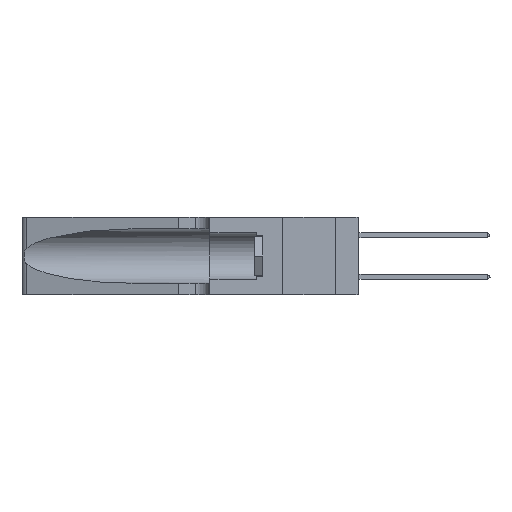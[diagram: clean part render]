
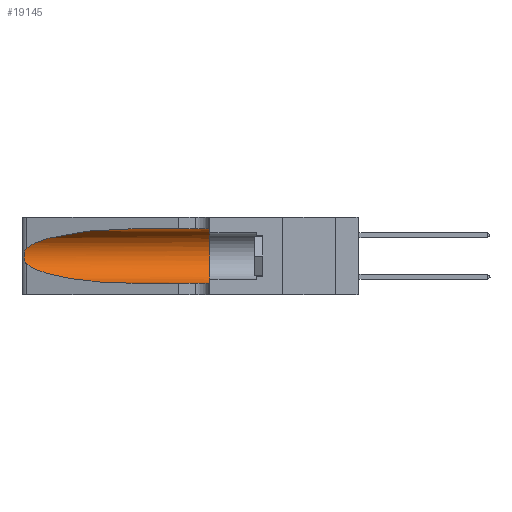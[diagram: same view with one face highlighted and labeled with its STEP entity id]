
A CAD part, left-side view. The second image highlights one B-rep face of the part: STEP entity #19145.
In plain terms, the highlighted cylindrical face has radius 3.308 mm (diameter 6.617 mm), a partial arc.
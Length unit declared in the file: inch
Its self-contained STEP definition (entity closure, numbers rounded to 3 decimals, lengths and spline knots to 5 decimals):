
#347 = EDGE_CURVE ( 'NONE', #3570, #11113, #22478, .T. ) ;
#1170 = CARTESIAN_POINT ( 'NONE',  ( 0.1305, 1.61858, 0.185 ) ) ;
#1408 = CARTESIAN_POINT ( 'NONE',  ( 0.1305, 0.72297, 0.05475 ) ) ;
#1459 = CIRCLE ( 'NONE', #18215, 0.13025 ) ;
#1961 = CARTESIAN_POINT ( 'NONE',  ( 0.25555, 1.22994, 0.2215 ) ) ;
#3570 = VERTEX_POINT ( 'NONE', #20307 ) ;
#3622 = DIRECTION ( 'NONE',  ( 0., -1., 0. ) ) ;
#4078 = DIRECTION ( 'NONE',  ( 0., 1., 0. ) ) ;
#4088 = CARTESIAN_POINT ( 'NONE',  ( 0.25787, 1.23484, 0.2124 ) ) ;
#4177 = CARTESIAN_POINT ( 'NONE',  ( 0.2373, 1.15595, 0.08982 ) ) ;
#4450 = CARTESIAN_POINT ( 'NONE',  ( 0.25639, 1.23186, 0.15144 ) ) ;
#4745 = CARTESIAN_POINT ( 'NONE',  ( 0.18966, 0.96281, 0.05475 ) ) ;
#5705 = CARTESIAN_POINT ( 'NONE',  ( 0.25487, 1.22718, 0.14631 ) ) ;
#5797 = ORIENTED_EDGE ( 'NONE', *, *, #26388, .T. ) ;
#5936 = ORIENTED_EDGE ( 'NONE', *, *, #347, .T. ) ;
#6123 = DIRECTION ( 'NONE',  ( 0., -1., 0. ) ) ;
#7045 = FACE_OUTER_BOUND ( 'NONE', #16669, .T. ) ;
#7656 = DIRECTION ( 'NONE',  ( 0., 0., -1. ) ) ;
#8499 = VERTEX_POINT ( 'NONE', #5705 ) ;
#8625 = CARTESIAN_POINT ( 'NONE',  ( 0.25555, 1.22993, 0.14849 ) ) ;
#8767 = CARTESIAN_POINT ( 'NONE',  ( 0.1305, 0.72297, 0.31525 ) ) ;
#9034 = CARTESIAN_POINT ( 'NONE',  ( 0.18966, 0.96281, 0.31525 ) ) ;
#9216 = ORIENTED_EDGE ( 'NONE', *, *, #14491, .T. ) ;
#10194 = CARTESIAN_POINT ( 'NONE',  ( 0.1305, 1.61858, 0.31525 ) ) ;
#10457 = ORIENTED_EDGE ( 'NONE', *, *, #23995, .F. ) ;
#10915 = CARTESIAN_POINT ( 'NONE',  ( 0.1305, 0.72297, 0.05475 ) ) ;
#11113 = VERTEX_POINT ( 'NONE', #25101 ) ;
#12879 = CARTESIAN_POINT ( 'NONE',  ( 0.26075, 1.23896, 0.19203 ) ) ;
#12976 = ORIENTED_EDGE ( 'NONE', *, *, #24922, .T. ) ;
#13323 = VERTEX_POINT ( 'NONE', #26771 ) ;
#13886 = VERTEX_POINT ( 'NONE', #10915 ) ;
#13900 = ORIENTED_EDGE ( 'NONE', *, *, #17628, .F. ) ;
#14491 = EDGE_CURVE ( 'NONE', #13886, #23960, #15539, .T. ) ;
#14859 = DIRECTION ( 'NONE',  ( 0., 0., 1. ) ) ;
#15539 = LINE ( 'NONE', #20869, #16569 ) ;
#16569 = VECTOR ( 'NONE', #3622, 39.37008 ) ;
#16669 = EDGE_LOOP ( 'NONE', ( #5936, #5797, #12976, #9216, #13900, #10457 ) ) ;
#16904 = CARTESIAN_POINT ( 'NONE',  ( 0.1305, 0.35, 0.05475 ) ) ;
#17628 = EDGE_CURVE ( 'NONE', #13323, #23960, #1459, .T. ) ;
#17926 = VECTOR ( 'NONE', #6123, 39.37008 ) ;
#18215 = AXIS2_PLACEMENT_3D ( 'NONE', #21323, #4078, #14859 ) ;
#18240 = DIRECTION ( 'NONE',  ( 0., -1., 0. ) ) ;
#19145 = ADVANCED_FACE ( 'NONE', ( #7045 ), #23695, .F. ) ;
#19330 = CARTESIAN_POINT ( 'NONE',  ( 0.25854, 1.2359, 0.20912 ) ) ;
#19411 = CARTESIAN_POINT ( 'NONE',  ( 0.26017, 1.23833, 0.17102 ) ) ;
#19871 =( BOUNDED_CURVE ( )  B_SPLINE_CURVE ( 3, ( #21605, #4177, #4745, #1408 ),
 .UNSPECIFIED., .F., .F. ) 
 B_SPLINE_CURVE_WITH_KNOTS ( ( 4, 4 ),
 ( 3.44316, 4.71239 ),
 .UNSPECIFIED. ) 
 CURVE ( )  GEOMETRIC_REPRESENTATION_ITEM ( )  RATIONAL_B_SPLINE_CURVE ( ( 1., 0.87, 0.87, 1. ) ) 
 REPRESENTATION_ITEM ( '' )  );
#20307 = CARTESIAN_POINT ( 'NONE',  ( 0.1305, 0.72297, 0.31525 ) ) ;
#20777 = B_SPLINE_CURVE_WITH_KNOTS ( 'NONE', 3,
 ( #25906, #1961, #23716, #4088, #19330, #21519, #12879, #28078, #19411, #21606, #21696, #4450, #8625, #25985 ),
 .UNSPECIFIED., .F., .F.,
 ( 4, 2, 2, 2, 2, 2, 4 ),
 ( 0., 0.00027, 0.00053, 0.00107, 0.0016, 0.00187, 0.00214 ),
 .UNSPECIFIED. ) ;
#20869 = CARTESIAN_POINT ( 'NONE',  ( 0.1305, 1.61858, 0.05475 ) ) ;
#21323 = CARTESIAN_POINT ( 'NONE',  ( 0.1305, 0.35, 0.185 ) ) ;
#21519 = CARTESIAN_POINT ( 'NONE',  ( 0.26018, 1.23835, 0.19895 ) ) ;
#21605 = CARTESIAN_POINT ( 'NONE',  ( 0.25487, 1.22718, 0.14631 ) ) ;
#21606 = CARTESIAN_POINT ( 'NONE',  ( 0.25856, 1.23593, 0.16098 ) ) ;
#21696 = CARTESIAN_POINT ( 'NONE',  ( 0.25789, 1.23486, 0.15765 ) ) ;
#22033 = LINE ( 'NONE', #10194, #17926 ) ;
#22478 =( BOUNDED_CURVE ( )  B_SPLINE_CURVE ( 3, ( #8767, #9034, #23944, #26128 ),
 .UNSPECIFIED., .F., .T. ) 
 B_SPLINE_CURVE_WITH_KNOTS ( ( 4, 4 ),
 ( 1.5708, 2.84003 ),
 .UNSPECIFIED. ) 
 CURVE ( )  GEOMETRIC_REPRESENTATION_ITEM ( )  RATIONAL_B_SPLINE_CURVE ( ( 1., 0.87, 0.87, 1. ) ) 
 REPRESENTATION_ITEM ( '' )  );
#23695 = CYLINDRICAL_SURFACE ( 'NONE', #25915, 0.13025 ) ;
#23716 = CARTESIAN_POINT ( 'NONE',  ( 0.25639, 1.23184, 0.21858 ) ) ;
#23944 = CARTESIAN_POINT ( 'NONE',  ( 0.2373, 1.15595, 0.28018 ) ) ;
#23960 = VERTEX_POINT ( 'NONE', #16904 ) ;
#23995 = EDGE_CURVE ( 'NONE', #3570, #13323, #22033, .T. ) ;
#24922 = EDGE_CURVE ( 'NONE', #8499, #13886, #19871, .T. ) ;
#25101 = CARTESIAN_POINT ( 'NONE',  ( 0.25487, 1.22718, 0.22369 ) ) ;
#25906 = CARTESIAN_POINT ( 'NONE',  ( 0.25487, 1.22718, 0.22369 ) ) ;
#25915 = AXIS2_PLACEMENT_3D ( 'NONE', #1170, #18240, #7656 ) ;
#25985 = CARTESIAN_POINT ( 'NONE',  ( 0.25487, 1.22718, 0.14631 ) ) ;
#26128 = CARTESIAN_POINT ( 'NONE',  ( 0.25487, 1.22718, 0.22369 ) ) ;
#26388 = EDGE_CURVE ( 'NONE', #11113, #8499, #20777, .T. ) ;
#26771 = CARTESIAN_POINT ( 'NONE',  ( 0.1305, 0.35, 0.31525 ) ) ;
#28078 = CARTESIAN_POINT ( 'NONE',  ( 0.26075, 1.23896, 0.178 ) ) ;
